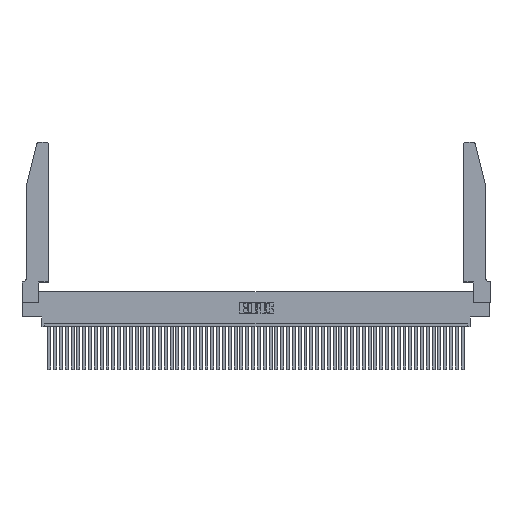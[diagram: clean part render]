
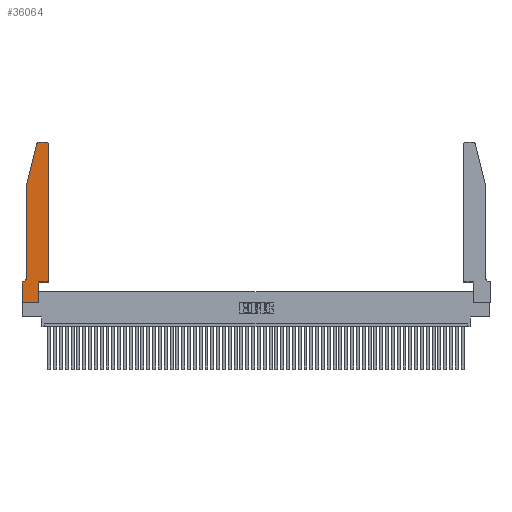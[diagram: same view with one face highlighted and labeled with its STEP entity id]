
A CAD part, top view. The second image highlights one B-rep face of the part: STEP entity #36064.
In plain terms, the highlighted planar face has unit normal (0, 0, 1).
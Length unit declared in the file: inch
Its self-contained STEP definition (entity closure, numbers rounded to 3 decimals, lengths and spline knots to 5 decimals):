
#1649 = ORIENTED_EDGE ( 'NONE', *, *, #7354, .T. ) ;
#1690 = VERTEX_POINT ( 'NONE', #37450 ) ;
#1977 = CARTESIAN_POINT ( 'NONE',  ( 0.4205, 2.75, 0.37 ) ) ;
#2018 = DIRECTION ( 'NONE',  ( -1., 0., 0. ) ) ;
#2221 = CARTESIAN_POINT ( 'NONE',  ( 0.284, 2.72, 0.37 ) ) ;
#3029 = CARTESIAN_POINT ( 'NONE',  ( 0., 0.35, 0.37 ) ) ;
#3255 = CARTESIAN_POINT ( 'NONE',  ( 0., 0.35, 0.37 ) ) ;
#3458 = CARTESIAN_POINT ( 'NONE',  ( 0.0755, 0.42, 0.37 ) ) ;
#3641 = CARTESIAN_POINT ( 'NONE',  ( 0.0055, 0.42, 0.37 ) ) ;
#3931 = LINE ( 'NONE', #48683, #27706 ) ;
#4395 = VERTEX_POINT ( 'NONE', #12202 ) ;
#4721 = VERTEX_POINT ( 'NONE', #27421 ) ;
#5527 = LINE ( 'NONE', #41408, #16822 ) ;
#5562 = VECTOR ( 'NONE', #41293, 39.37008 ) ;
#6038 = CARTESIAN_POINT ( 'NONE',  ( 0.4205, 2.72, 0.37 ) ) ;
#6753 = DIRECTION ( 'NONE',  ( 0., 0., 1. ) ) ;
#7019 = LINE ( 'NONE', #53922, #5562 ) ;
#7354 = EDGE_CURVE ( 'NONE', #7711, #4395, #11526, .T. ) ;
#7561 = LINE ( 'NONE', #12581, #10149 ) ;
#7711 = VERTEX_POINT ( 'NONE', #28005 ) ;
#7762 = DIRECTION ( 'NONE',  ( 0., 1., 0. ) ) ;
#7927 = DIRECTION ( 'NONE',  ( -1., 0., 0. ) ) ;
#8186 = VERTEX_POINT ( 'NONE', #9840 ) ;
#8389 = EDGE_CURVE ( 'NONE', #21781, #8186, #16753, .T. ) ;
#8977 = CARTESIAN_POINT ( 'NONE',  ( 0., 0., 0.37 ) ) ;
#9840 = CARTESIAN_POINT ( 'NONE',  ( 0.0055, 0.35, 0.37 ) ) ;
#10149 = VECTOR ( 'NONE', #21751, 39.37008 ) ;
#10904 = VERTEX_POINT ( 'NONE', #3255 ) ;
#11526 = LINE ( 'NONE', #11581, #34582 ) ;
#11581 = CARTESIAN_POINT ( 'NONE',  ( 0.4505, 0.35, 0.37 ) ) ;
#11847 = LINE ( 'NONE', #8977, #25074 ) ;
#11876 = CIRCLE ( 'NONE', #12867, 0.03 ) ;
#12202 = CARTESIAN_POINT ( 'NONE',  ( 0.4505, 0.35, 0.37 ) ) ;
#12581 = CARTESIAN_POINT ( 'NONE',  ( 0.2605, 2.75, 0.37 ) ) ;
#12867 = AXIS2_PLACEMENT_3D ( 'NONE', #6038, #22575, #31707 ) ;
#12877 = EDGE_CURVE ( 'NONE', #24023, #46563, #7019, .T. ) ;
#13525 = CIRCLE ( 'NONE', #49105, 0.03 ) ;
#13561 = ORIENTED_EDGE ( 'NONE', *, *, #27006, .T. ) ;
#16077 = AXIS2_PLACEMENT_3D ( 'NONE', #3029, #6753, #19670 ) ;
#16753 = CIRCLE ( 'NONE', #49804, 0.07 ) ;
#16822 = VECTOR ( 'NONE', #7762, 39.37008 ) ;
#17898 = VECTOR ( 'NONE', #29151, 39.37008 ) ;
#18334 = CARTESIAN_POINT ( 'NONE',  ( 0.4505, 0.35, 0.37 ) ) ;
#19670 = DIRECTION ( 'NONE',  ( 1., 0., 0. ) ) ;
#20039 = ORIENTED_EDGE ( 'NONE', *, *, #39453, .T. ) ;
#21751 = DIRECTION ( 'NONE',  ( -1., 0., 0. ) ) ;
#21781 = VERTEX_POINT ( 'NONE', #3458 ) ;
#22575 = DIRECTION ( 'NONE',  ( 0., 0., 1. ) ) ;
#22962 = ORIENTED_EDGE ( 'NONE', *, *, #52996, .T. ) ;
#23675 = VERTEX_POINT ( 'NONE', #34827 ) ;
#23855 = VERTEX_POINT ( 'NONE', #1977 ) ;
#24023 = VERTEX_POINT ( 'NONE', #25997 ) ;
#24278 = PLANE ( 'NONE',  #16077 ) ;
#24850 = DIRECTION ( 'NONE',  ( 1., 0., 0. ) ) ;
#25074 = VECTOR ( 'NONE', #33911, 39.37008 ) ;
#25491 = EDGE_CURVE ( 'NONE', #4721, #23855, #11876, .T. ) ;
#25997 = CARTESIAN_POINT ( 'NONE',  ( 0., 0., 0.37 ) ) ;
#26632 = ORIENTED_EDGE ( 'NONE', *, *, #28040, .T. ) ;
#27006 = EDGE_CURVE ( 'NONE', #46563, #7711, #5527, .T. ) ;
#27421 = CARTESIAN_POINT ( 'NONE',  ( 0.4505, 2.72, 0.37 ) ) ;
#27706 = VECTOR ( 'NONE', #2018, 39.37008 ) ;
#28005 = CARTESIAN_POINT ( 'NONE',  ( 0.2865, 0.35, 0.37 ) ) ;
#28040 = EDGE_CURVE ( 'NONE', #1690, #21781, #49790, .T. ) ;
#28986 = CARTESIAN_POINT ( 'NONE',  ( 0.2865, 0., 0.37 ) ) ;
#29151 = DIRECTION ( 'NONE',  ( 0., -1., 0. ) ) ;
#29804 = ORIENTED_EDGE ( 'NONE', *, *, #35084, .T. ) ;
#30485 = ORIENTED_EDGE ( 'NONE', *, *, #25491, .T. ) ;
#31707 = DIRECTION ( 'NONE',  ( 1., 0., 0. ) ) ;
#31885 = ORIENTED_EDGE ( 'NONE', *, *, #40320, .T. ) ;
#32811 = LINE ( 'NONE', #53412, #41456 ) ;
#33207 = DIRECTION ( 'NONE',  ( 0., 0., -1. ) ) ;
#33567 = ORIENTED_EDGE ( 'NONE', *, *, #12877, .T. ) ;
#33911 = DIRECTION ( 'NONE',  ( 0., -1., 0. ) ) ;
#34430 = EDGE_CURVE ( 'NONE', #23675, #1690, #32811, .T. ) ;
#34582 = VECTOR ( 'NONE', #24850, 39.37008 ) ;
#34827 = CARTESIAN_POINT ( 'NONE',  ( 0.25487, 2.72718, 0.37 ) ) ;
#35084 = EDGE_CURVE ( 'NONE', #4395, #4721, #40666, .T. ) ;
#35341 = EDGE_LOOP ( 'NONE', ( #31885, #20039, #46936, #26632, #42752, #38589, #22962, #33567, #13561, #1649, #29804, #30485 ) ) ;
#35677 = DIRECTION ( 'NONE',  ( 1., 0., 0. ) ) ;
#36064 = ADVANCED_FACE ( 'NONE', ( #51122 ), #24278, .T. ) ;
#36074 = DIRECTION ( 'NONE',  ( 0., 0., 1. ) ) ;
#37450 = CARTESIAN_POINT ( 'NONE',  ( 0.0755, 2., 0.37 ) ) ;
#38010 = VECTOR ( 'NONE', #52020, 39.37008 ) ;
#38589 = ORIENTED_EDGE ( 'NONE', *, *, #51042, .T. ) ;
#39139 = VERTEX_POINT ( 'NONE', #41619 ) ;
#39453 = EDGE_CURVE ( 'NONE', #39139, #23675, #13525, .T. ) ;
#40320 = EDGE_CURVE ( 'NONE', #23855, #39139, #7561, .T. ) ;
#40666 = LINE ( 'NONE', #18334, #38010 ) ;
#40799 = DIRECTION ( 'NONE',  ( -0.239, -0.971, 0. ) ) ;
#41293 = DIRECTION ( 'NONE',  ( 1., 0., 0. ) ) ;
#41380 = CARTESIAN_POINT ( 'NONE',  ( 0.0755, 2., 0.37 ) ) ;
#41408 = CARTESIAN_POINT ( 'NONE',  ( 0.2865, 0.35, 0.37 ) ) ;
#41456 = VECTOR ( 'NONE', #40799, 39.37008 ) ;
#41619 = CARTESIAN_POINT ( 'NONE',  ( 0.284, 2.75, 0.37 ) ) ;
#42752 = ORIENTED_EDGE ( 'NONE', *, *, #8389, .T. ) ;
#46563 = VERTEX_POINT ( 'NONE', #28986 ) ;
#46936 = ORIENTED_EDGE ( 'NONE', *, *, #34430, .T. ) ;
#48683 = CARTESIAN_POINT ( 'NONE',  ( 0.0755, 0.35, 0.37 ) ) ;
#49105 = AXIS2_PLACEMENT_3D ( 'NONE', #2221, #36074, #35677 ) ;
#49790 = LINE ( 'NONE', #41380, #17898 ) ;
#49804 = AXIS2_PLACEMENT_3D ( 'NONE', #3641, #33207, #7927 ) ;
#51042 = EDGE_CURVE ( 'NONE', #8186, #10904, #3931, .T. ) ;
#51122 = FACE_OUTER_BOUND ( 'NONE', #35341, .T. ) ;
#52020 = DIRECTION ( 'NONE',  ( 0., 1., 0. ) ) ;
#52996 = EDGE_CURVE ( 'NONE', #10904, #24023, #11847, .T. ) ;
#53412 = CARTESIAN_POINT ( 'NONE',  ( 0.0755, 2., 0.37 ) ) ;
#53922 = CARTESIAN_POINT ( 'NONE',  ( 0., 0., 0.37 ) ) ;
